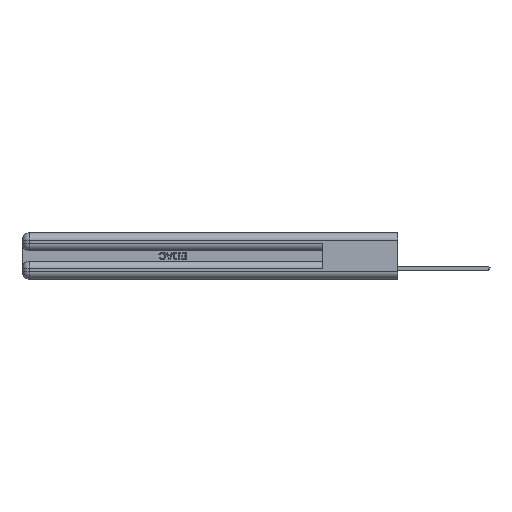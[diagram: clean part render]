
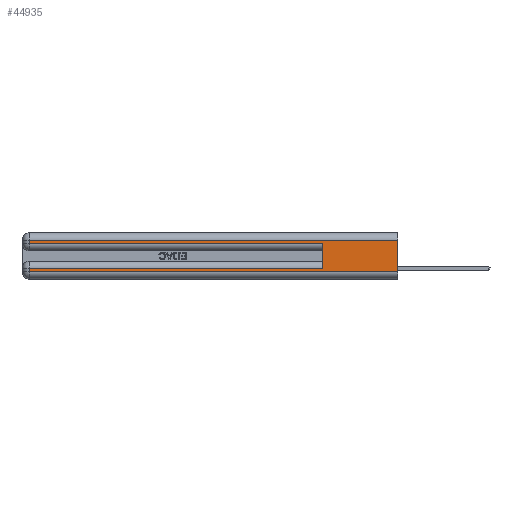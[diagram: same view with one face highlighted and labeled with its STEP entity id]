
A CAD part, left-side view. The second image highlights one B-rep face of the part: STEP entity #44935.
In plain terms, the highlighted planar face has unit normal (-1, 0, 0).
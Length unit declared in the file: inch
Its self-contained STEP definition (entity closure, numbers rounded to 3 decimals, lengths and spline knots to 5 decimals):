
#2929 = CARTESIAN_POINT ( 'NONE',  ( 0., 2.94, 0.06 ) ) ;
#3159 = DIRECTION ( 'NONE',  ( 0., -1., 0. ) ) ;
#4050 = EDGE_CURVE ( 'NONE', #4054, #33165, #39528, .T. ) ;
#4054 = VERTEX_POINT ( 'NONE', #31993 ) ;
#5223 = EDGE_CURVE ( 'NONE', #23586, #29734, #31982, .T. ) ;
#5626 = LINE ( 'NONE', #8360, #6169 ) ;
#5727 = EDGE_CURVE ( 'NONE', #4054, #7221, #7538, .T. ) ;
#6053 = EDGE_CURVE ( 'NONE', #23586, #36437, #9823, .T. ) ;
#6068 = DIRECTION ( 'NONE',  ( 1., 0., 0. ) ) ;
#6169 = VECTOR ( 'NONE', #15482, 39.37008 ) ;
#6239 = ORIENTED_EDGE ( 'NONE', *, *, #8306, .T. ) ;
#6461 = VECTOR ( 'NONE', #8855, 39.37008 ) ;
#6597 = DIRECTION ( 'NONE',  ( 0., 1., 0. ) ) ;
#7177 = VERTEX_POINT ( 'NONE', #2929 ) ;
#7221 = VERTEX_POINT ( 'NONE', #35510 ) ;
#7538 = LINE ( 'NONE', #9131, #30786 ) ;
#8306 = EDGE_CURVE ( 'NONE', #29734, #14635, #5626, .T. ) ;
#8360 = CARTESIAN_POINT ( 'NONE',  ( 0., 2.94, 0.37 ) ) ;
#8495 = DIRECTION ( 'NONE',  ( 0., 0., 1. ) ) ;
#8855 = DIRECTION ( 'NONE',  ( 0., 0., -1. ) ) ;
#9131 = CARTESIAN_POINT ( 'NONE',  ( 0., 0.6, 0.145 ) ) ;
#9701 = ORIENTED_EDGE ( 'NONE', *, *, #4050, .T. ) ;
#9823 = LINE ( 'NONE', #21795, #32489 ) ;
#10291 = EDGE_CURVE ( 'NONE', #33165, #7177, #40027, .T. ) ;
#11859 = VECTOR ( 'NONE', #3159, 39.37008 ) ;
#13115 = CARTESIAN_POINT ( 'NONE',  ( 0., 0., 0.31 ) ) ;
#13976 = LINE ( 'NONE', #29017, #27623 ) ;
#14331 = VECTOR ( 'NONE', #45394, 39.37008 ) ;
#14472 = VECTOR ( 'NONE', #6597, 39.37008 ) ;
#14482 = EDGE_LOOP ( 'NONE', ( #30833, #44192, #6239, #38790, #14878, #9701, #34659, #35212 ) ) ;
#14635 = VERTEX_POINT ( 'NONE', #15453 ) ;
#14878 = ORIENTED_EDGE ( 'NONE', *, *, #5727, .F. ) ;
#15453 = CARTESIAN_POINT ( 'NONE',  ( 0., 2.94, 0.285 ) ) ;
#15482 = DIRECTION ( 'NONE',  ( 0., 0., -1. ) ) ;
#15962 = CARTESIAN_POINT ( 'NONE',  ( 0., 2.94, 0.37 ) ) ;
#17478 = CARTESIAN_POINT ( 'NONE',  ( 0., 0., 0.06 ) ) ;
#18076 = CARTESIAN_POINT ( 'NONE',  ( 0., 0., 0.285 ) ) ;
#20345 = DIRECTION ( 'NONE',  ( 0., 0., -1. ) ) ;
#21795 = CARTESIAN_POINT ( 'NONE',  ( 0., 0., 0.37 ) ) ;
#23377 = CARTESIAN_POINT ( 'NONE',  ( 0., 0., 0.31 ) ) ;
#23586 = VERTEX_POINT ( 'NONE', #23377 ) ;
#24125 = CARTESIAN_POINT ( 'NONE',  ( 0., 2.94, 0.085 ) ) ;
#27623 = VECTOR ( 'NONE', #33286, 39.37008 ) ;
#27819 = CARTESIAN_POINT ( 'NONE',  ( 0., 2.94, 0.31 ) ) ;
#28347 = CARTESIAN_POINT ( 'NONE',  ( 0., 0., 0.085 ) ) ;
#29017 = CARTESIAN_POINT ( 'NONE',  ( 0., 0., 0.06 ) ) ;
#29734 = VERTEX_POINT ( 'NONE', #27819 ) ;
#30786 = VECTOR ( 'NONE', #8495, 39.37008 ) ;
#30833 = ORIENTED_EDGE ( 'NONE', *, *, #6053, .F. ) ;
#30994 = PLANE ( 'NONE',  #36881 ) ;
#31982 = LINE ( 'NONE', #13115, #14331 ) ;
#31993 = CARTESIAN_POINT ( 'NONE',  ( 0., 0.6, 0.085 ) ) ;
#32489 = VECTOR ( 'NONE', #43734, 39.37008 ) ;
#33165 = VERTEX_POINT ( 'NONE', #24125 ) ;
#33286 = DIRECTION ( 'NONE',  ( 0., -1., 0. ) ) ;
#34659 = ORIENTED_EDGE ( 'NONE', *, *, #10291, .T. ) ;
#35212 = ORIENTED_EDGE ( 'NONE', *, *, #37305, .T. ) ;
#35510 = CARTESIAN_POINT ( 'NONE',  ( 0., 0.6, 0.285 ) ) ;
#35742 = EDGE_CURVE ( 'NONE', #14635, #7221, #45990, .T. ) ;
#36437 = VERTEX_POINT ( 'NONE', #17478 ) ;
#36881 = AXIS2_PLACEMENT_3D ( 'NONE', #38788, #6068, #20345 ) ;
#37305 = EDGE_CURVE ( 'NONE', #7177, #36437, #13976, .T. ) ;
#37720 = FACE_OUTER_BOUND ( 'NONE', #14482, .T. ) ;
#38788 = CARTESIAN_POINT ( 'NONE',  ( 0., 0., 0.37 ) ) ;
#38790 = ORIENTED_EDGE ( 'NONE', *, *, #35742, .T. ) ;
#39528 = LINE ( 'NONE', #28347, #14472 ) ;
#40027 = LINE ( 'NONE', #15962, #6461 ) ;
#43734 = DIRECTION ( 'NONE',  ( 0., 0., -1. ) ) ;
#44192 = ORIENTED_EDGE ( 'NONE', *, *, #5223, .T. ) ;
#44935 = ADVANCED_FACE ( 'NONE', ( #37720 ), #30994, .F. ) ;
#45394 = DIRECTION ( 'NONE',  ( 0., 1., 0. ) ) ;
#45990 = LINE ( 'NONE', #18076, #11859 ) ;
